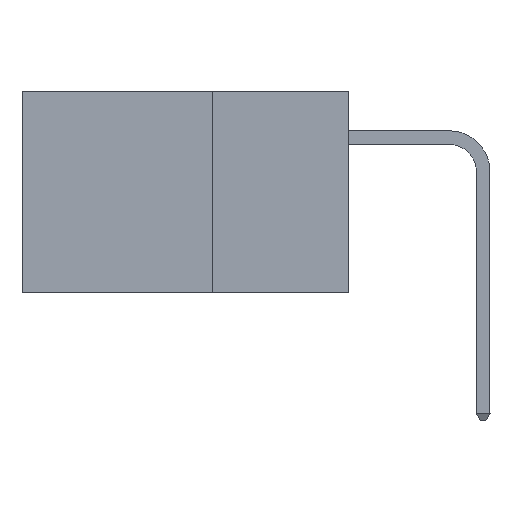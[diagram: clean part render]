
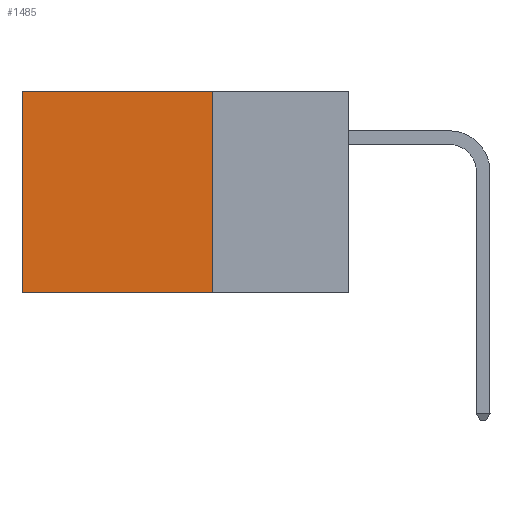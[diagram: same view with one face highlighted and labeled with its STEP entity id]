
A CAD part, left-side view. The second image highlights one B-rep face of the part: STEP entity #1485.
In plain terms, the highlighted planar face has unit normal (-1, 0, 0).
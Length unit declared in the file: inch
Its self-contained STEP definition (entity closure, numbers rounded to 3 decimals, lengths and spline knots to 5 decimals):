
#117 = ORIENTED_EDGE ( 'NONE', *, *, #2382, .T. ) ;
#551 = DIRECTION ( 'NONE',  ( 0., 1., 0. ) ) ;
#1245 = ORIENTED_EDGE ( 'NONE', *, *, #11637, .F. ) ;
#1473 = VECTOR ( 'NONE', #8938, 39.37008 ) ;
#1485 = ADVANCED_FACE ( 'NONE', ( #11789 ), #7357, .F. ) ;
#1608 = LINE ( 'NONE', #10749, #11269 ) ;
#2235 = CARTESIAN_POINT ( 'NONE',  ( 0.2875, 0.25, -0.37 ) ) ;
#2382 = EDGE_CURVE ( 'NONE', #10943, #5857, #10828, .T. ) ;
#3729 = CARTESIAN_POINT ( 'NONE',  ( 0.2875, 0.25, -0.37 ) ) ;
#3911 = DIRECTION ( 'NONE',  ( 0., 0., -1. ) ) ;
#4513 = LINE ( 'NONE', #11270, #1473 ) ;
#5857 = VERTEX_POINT ( 'NONE', #8561 ) ;
#6157 = CARTESIAN_POINT ( 'NONE',  ( 0.2875, 0.25, 0. ) ) ;
#6463 = AXIS2_PLACEMENT_3D ( 'NONE', #6157, #10806, #3911 ) ;
#7357 = PLANE ( 'NONE',  #6463 ) ;
#7691 = EDGE_CURVE ( 'NONE', #10943, #12806, #4513, .T. ) ;
#7728 = CARTESIAN_POINT ( 'NONE',  ( 0.2875, 0.25, 0. ) ) ;
#7792 = ORIENTED_EDGE ( 'NONE', *, *, #13341, .T. ) ;
#8299 = VERTEX_POINT ( 'NONE', #11703 ) ;
#8561 = CARTESIAN_POINT ( 'NONE',  ( 0.2875, 0.6, 0. ) ) ;
#8645 = DIRECTION ( 'NONE',  ( 0., 1., 0. ) ) ;
#8938 = DIRECTION ( 'NONE',  ( 0., 0., -1. ) ) ;
#10619 = LINE ( 'NONE', #3729, #12917 ) ;
#10749 = CARTESIAN_POINT ( 'NONE',  ( 0.2875, 0.6, 0. ) ) ;
#10806 = DIRECTION ( 'NONE',  ( 1., 0., 0. ) ) ;
#10828 = LINE ( 'NONE', #10970, #11133 ) ;
#10943 = VERTEX_POINT ( 'NONE', #7728 ) ;
#10970 = CARTESIAN_POINT ( 'NONE',  ( 0.2875, 0.25, 0. ) ) ;
#11133 = VECTOR ( 'NONE', #8645, 39.37008 ) ;
#11269 = VECTOR ( 'NONE', #13078, 39.37008 ) ;
#11270 = CARTESIAN_POINT ( 'NONE',  ( 0.2875, 0.25, 0. ) ) ;
#11637 = EDGE_CURVE ( 'NONE', #12806, #8299, #10619, .T. ) ;
#11703 = CARTESIAN_POINT ( 'NONE',  ( 0.2875, 0.6, -0.37 ) ) ;
#11710 = EDGE_LOOP ( 'NONE', ( #7792, #1245, #13697, #117 ) ) ;
#11789 = FACE_OUTER_BOUND ( 'NONE', #11710, .T. ) ;
#12806 = VERTEX_POINT ( 'NONE', #2235 ) ;
#12917 = VECTOR ( 'NONE', #551, 39.37008 ) ;
#13078 = DIRECTION ( 'NONE',  ( 0., 0., -1. ) ) ;
#13341 = EDGE_CURVE ( 'NONE', #5857, #8299, #1608, .T. ) ;
#13697 = ORIENTED_EDGE ( 'NONE', *, *, #7691, .F. ) ;
